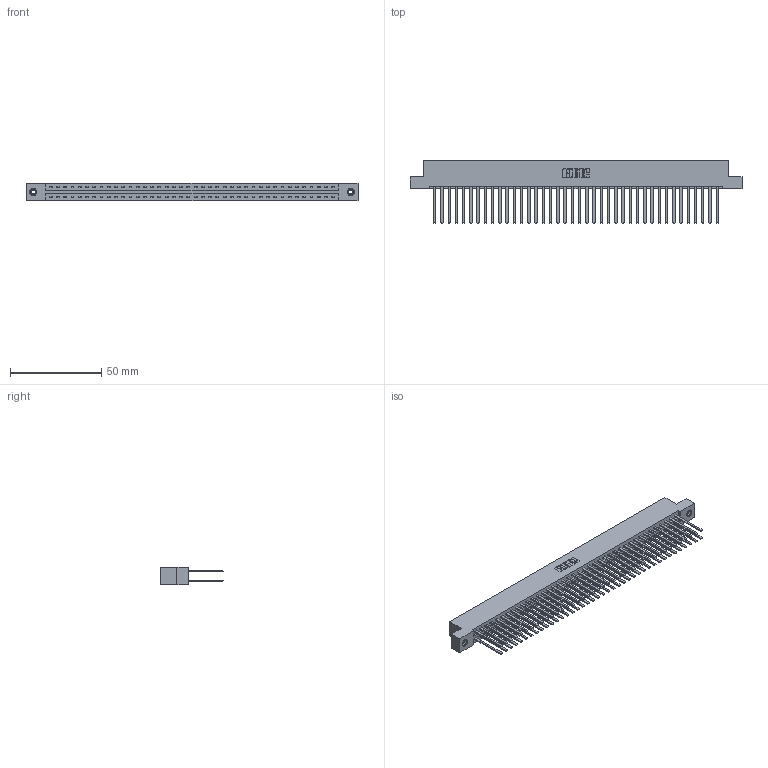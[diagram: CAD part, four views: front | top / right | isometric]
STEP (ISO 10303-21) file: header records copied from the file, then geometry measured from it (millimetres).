
FILE_DESCRIPTION (( 'STEP AP203' ), '1' );
FILE_NAME ('337-080-544-208.STEP', '2018-08-12T18:25:05', ( '' ), ( '' ), 'SwSTEP 2.0', 'SolidWorks 2016', '' );
FILE_SCHEMA (( 'CONFIG_CONTROL_DESIGN' ));
Length unit declared in the file: inch
Products named in the file (4): 337 Part_Flush Mounting Lugs - 0.156 Dia-TI; 345-292-001_345-293-144; 345-250-001_345-250-003-102; 337-080-544-208
Assembly tree (83 placements, depth 2):
  337-080-544-208
    337 Part_Flush Mounting Lugs - 0.156 Dia-TI
    345-292-001_345-293-144  x80
    345-250-001_345-250-003-102  x2
Bounding box: 181.51 x 34.3 x 9.4 mm (x, y, z)
Volume: 20217.1 mm3; surface area: 26523.5 mm2
Topology: 83 solids, 83 shells, 4014 faces, 11887 edges, 7810 vertices
Faces by surface type: plane 2822, cylinder 1176, cone 12, torus 4
Entity records: 32274 total; most frequent: CARTESIAN_POINT 5417, ORIENTED_EDGE 5346, DIRECTION 4639, EDGE_CURVE 2673, VECTOR 2529, LINE 2529, VERTEX_POINT 1776, AXIS2_PLACEMENT_3D 1055
